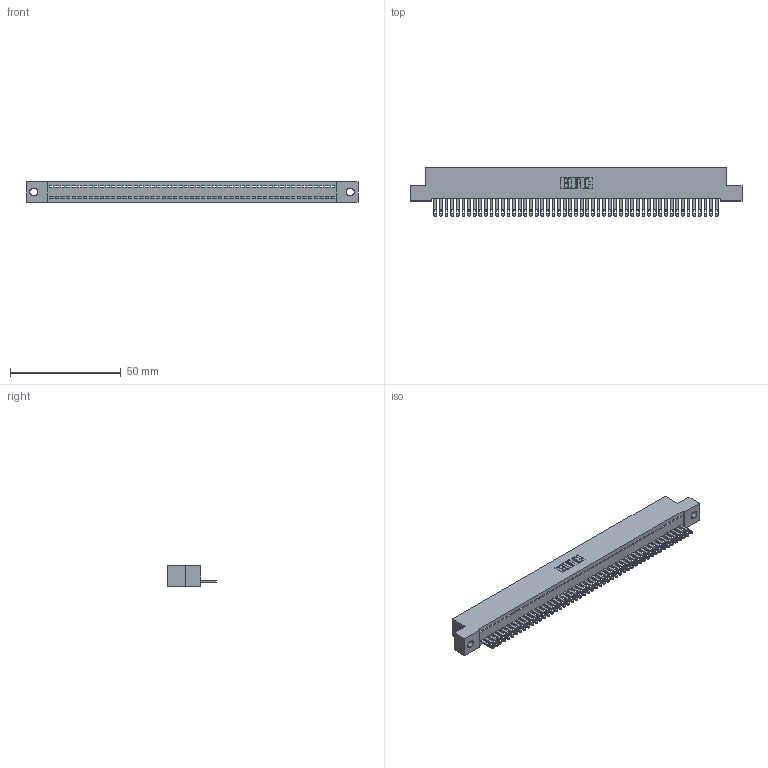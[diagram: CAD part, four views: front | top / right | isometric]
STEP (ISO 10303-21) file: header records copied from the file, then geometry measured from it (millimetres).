
FILE_DESCRIPTION (( 'STEP AP203' ), '1' );
FILE_NAME ('892-051-500-102.STEP', '2020-09-21T17:55:57', ( '' ), ( '' ), 'SwSTEP 2.0', 'SolidWorks 2020', '' );
FILE_SCHEMA (( 'CONFIG_CONTROL_DESIGN' ));
Length unit declared in the file: inch
Products named in the file (3): 892-051-500-102; 345-292-001_345-293-100; 842 Part_.128 Slot
Assembly tree (52 placements, depth 2):
  892-051-500-102
    842 Part_.128 Slot
    345-292-001_345-293-100  x51
Bounding box: 149.86 x 21.85 x 9.4 mm (x, y, z)
Volume: 13152.3 mm3; surface area: 19341.6 mm2
Topology: 52 solids, 52 shells, 2868 faces, 8879 edges, 5918 vertices
Faces by surface type: plane 1906, cylinder 962
Entity records: 29947 total; most frequent: CARTESIAN_POINT 5171, ORIENTED_EDGE 5158, DIRECTION 4345, EDGE_CURVE 2579, LINE 2447, VECTOR 2447, VERTEX_POINT 1718, AXIS2_PLACEMENT_3D 949
